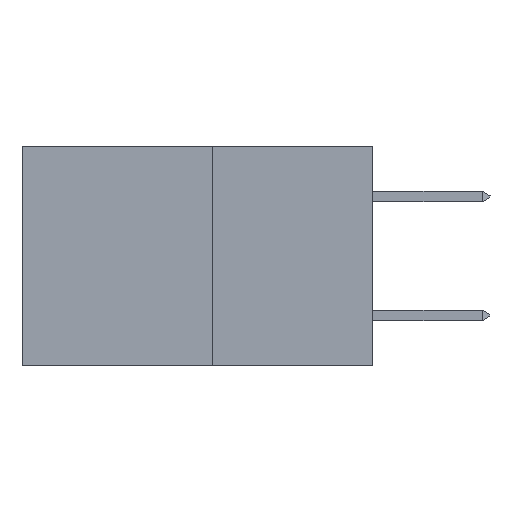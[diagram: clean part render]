
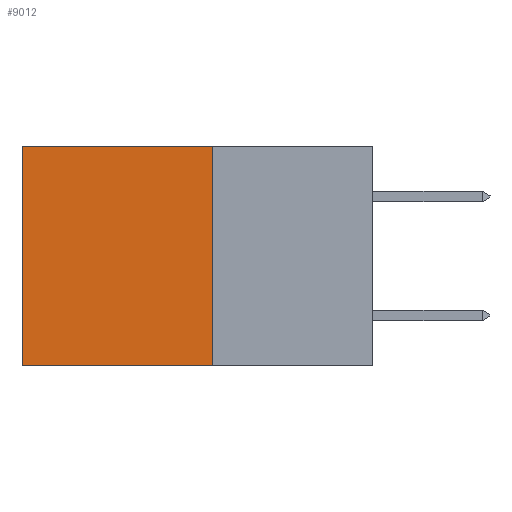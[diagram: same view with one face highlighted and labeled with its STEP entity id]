
A CAD part, left-side view. The second image highlights one B-rep face of the part: STEP entity #9012.
In plain terms, the highlighted planar face has unit normal (-1, 0, 0).
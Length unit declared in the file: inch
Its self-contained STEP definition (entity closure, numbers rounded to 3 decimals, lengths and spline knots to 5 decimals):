
#274 = VECTOR ( 'NONE', #7711, 39.37008 ) ;
#543 = DIRECTION ( 'NONE',  ( 0., 0., -1. ) ) ;
#1467 = EDGE_CURVE ( 'NONE', #7746, #7793, #3886, .T. ) ;
#1798 = DIRECTION ( 'NONE',  ( 0., 0., -1. ) ) ;
#1893 = VECTOR ( 'NONE', #1798, 39.37008 ) ;
#2002 = VERTEX_POINT ( 'NONE', #9443 ) ;
#2083 = LINE ( 'NONE', #7739, #274 ) ;
#2440 = VECTOR ( 'NONE', #4793, 39.37008 ) ;
#2606 = DIRECTION ( 'NONE',  ( 0., 1., 0. ) ) ;
#2838 = ORIENTED_EDGE ( 'NONE', *, *, #5320, .T. ) ;
#2875 = AXIS2_PLACEMENT_3D ( 'NONE', #7217, #5060, #543 ) ;
#2895 = LINE ( 'NONE', #4982, #2440 ) ;
#3328 = LINE ( 'NONE', #8461, #5324 ) ;
#3886 = LINE ( 'NONE', #5793, #1893 ) ;
#4320 = PLANE ( 'NONE',  #2875 ) ;
#4557 = CARTESIAN_POINT ( 'NONE',  ( 0.277, 0.59, 0. ) ) ;
#4604 = ORIENTED_EDGE ( 'NONE', *, *, #7980, .F. ) ;
#4667 = EDGE_LOOP ( 'NONE', ( #6126, #4604, #8216, #2838 ) ) ;
#4793 = DIRECTION ( 'NONE',  ( 0., 1., 0. ) ) ;
#4982 = CARTESIAN_POINT ( 'NONE',  ( 0.277, 0.27, 0. ) ) ;
#5060 = DIRECTION ( 'NONE',  ( 1., 0., 0. ) ) ;
#5108 = EDGE_CURVE ( 'NONE', #2002, #7209, #2083, .T. ) ;
#5320 = EDGE_CURVE ( 'NONE', #2002, #7746, #2895, .T. ) ;
#5324 = VECTOR ( 'NONE', #2606, 39.37008 ) ;
#5632 = FACE_OUTER_BOUND ( 'NONE', #4667, .T. ) ;
#5793 = CARTESIAN_POINT ( 'NONE',  ( 0.277, 0.59, -0.37 ) ) ;
#6126 = ORIENTED_EDGE ( 'NONE', *, *, #1467, .T. ) ;
#6830 = CARTESIAN_POINT ( 'NONE',  ( 0.277, 0.59, -0.37 ) ) ;
#7209 = VERTEX_POINT ( 'NONE', #7430 ) ;
#7217 = CARTESIAN_POINT ( 'NONE',  ( 0.277, 0.27, -0.37 ) ) ;
#7430 = CARTESIAN_POINT ( 'NONE',  ( 0.277, 0.27, -0.37 ) ) ;
#7711 = DIRECTION ( 'NONE',  ( 0., 0., -1. ) ) ;
#7739 = CARTESIAN_POINT ( 'NONE',  ( 0.277, 0.27, -0.37 ) ) ;
#7746 = VERTEX_POINT ( 'NONE', #4557 ) ;
#7793 = VERTEX_POINT ( 'NONE', #6830 ) ;
#7980 = EDGE_CURVE ( 'NONE', #7209, #7793, #3328, .T. ) ;
#8216 = ORIENTED_EDGE ( 'NONE', *, *, #5108, .F. ) ;
#8461 = CARTESIAN_POINT ( 'NONE',  ( 0.277, 0.27, -0.37 ) ) ;
#9012 = ADVANCED_FACE ( 'NONE', ( #5632 ), #4320, .F. ) ;
#9443 = CARTESIAN_POINT ( 'NONE',  ( 0.277, 0.27, 0. ) ) ;
